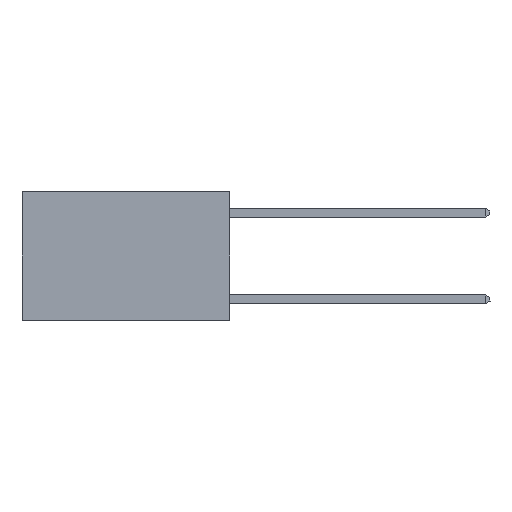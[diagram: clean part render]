
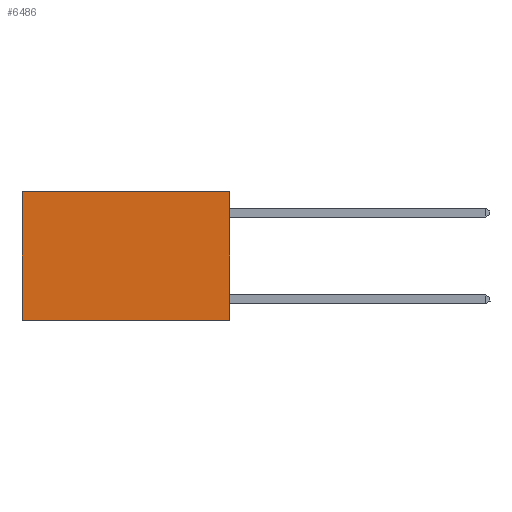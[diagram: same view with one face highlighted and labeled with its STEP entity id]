
A CAD part, left-side view. The second image highlights one B-rep face of the part: STEP entity #6486.
In plain terms, the highlighted planar face has unit normal (-1, 0, 0).
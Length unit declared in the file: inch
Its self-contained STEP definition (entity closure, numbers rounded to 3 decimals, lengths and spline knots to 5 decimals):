
#90 = LINE ( 'NONE', #4527, #2439 ) ;
#197 = FACE_OUTER_BOUND ( 'NONE', #1387, .T. ) ;
#447 = VECTOR ( 'NONE', #11134, 39.37008 ) ;
#1387 = EDGE_LOOP ( 'NONE', ( #4342, #4482, #4701, #6174 ) ) ;
#1557 = EDGE_CURVE ( 'NONE', #8174, #9598, #2624, .T. ) ;
#2381 = CARTESIAN_POINT ( 'NONE',  ( 0.2625, 0., -0.37 ) ) ;
#2439 = VECTOR ( 'NONE', #4556, 39.37008 ) ;
#2540 = CARTESIAN_POINT ( 'NONE',  ( 0.2625, 0.6, -0.37 ) ) ;
#2624 = LINE ( 'NONE', #2381, #8128 ) ;
#2649 = DIRECTION ( 'NONE',  ( 0., 1., 0. ) ) ;
#2744 = EDGE_CURVE ( 'NONE', #10024, #9598, #90, .T. ) ;
#2988 = CARTESIAN_POINT ( 'NONE',  ( 0.2625, 0.6, 0. ) ) ;
#3643 = CARTESIAN_POINT ( 'NONE',  ( 0.2625, 0., 0. ) ) ;
#4246 = VERTEX_POINT ( 'NONE', #7286 ) ;
#4342 = ORIENTED_EDGE ( 'NONE', *, *, #2744, .T. ) ;
#4482 = ORIENTED_EDGE ( 'NONE', *, *, #1557, .F. ) ;
#4527 = CARTESIAN_POINT ( 'NONE',  ( 0.2625, 0.6, 0. ) ) ;
#4556 = DIRECTION ( 'NONE',  ( 0., 0., -1. ) ) ;
#4654 = DIRECTION ( 'NONE',  ( 0., 0., -1. ) ) ;
#4701 = ORIENTED_EDGE ( 'NONE', *, *, #11462, .F. ) ;
#5405 = CARTESIAN_POINT ( 'NONE',  ( 0.2625, 0., -0.37 ) ) ;
#6023 = LINE ( 'NONE', #10167, #447 ) ;
#6174 = ORIENTED_EDGE ( 'NONE', *, *, #6508, .T. ) ;
#6486 = ADVANCED_FACE ( 'NONE', ( #197 ), #9510, .F. ) ;
#6508 = EDGE_CURVE ( 'NONE', #4246, #10024, #9743, .T. ) ;
#6650 = DIRECTION ( 'NONE',  ( 0., 1., 0. ) ) ;
#7286 = CARTESIAN_POINT ( 'NONE',  ( 0.2625, 0., 0. ) ) ;
#7859 = AXIS2_PLACEMENT_3D ( 'NONE', #3643, #10503, #4654 ) ;
#8128 = VECTOR ( 'NONE', #2649, 39.37008 ) ;
#8174 = VERTEX_POINT ( 'NONE', #5405 ) ;
#9510 = PLANE ( 'NONE',  #7859 ) ;
#9598 = VERTEX_POINT ( 'NONE', #2540 ) ;
#9743 = LINE ( 'NONE', #11463, #12004 ) ;
#10024 = VERTEX_POINT ( 'NONE', #2988 ) ;
#10167 = CARTESIAN_POINT ( 'NONE',  ( 0.2625, 0., 0. ) ) ;
#10503 = DIRECTION ( 'NONE',  ( 1., 0., 0. ) ) ;
#11134 = DIRECTION ( 'NONE',  ( 0., 0., -1. ) ) ;
#11462 = EDGE_CURVE ( 'NONE', #4246, #8174, #6023, .T. ) ;
#11463 = CARTESIAN_POINT ( 'NONE',  ( 0.2625, 0., 0. ) ) ;
#12004 = VECTOR ( 'NONE', #6650, 39.37008 ) ;
